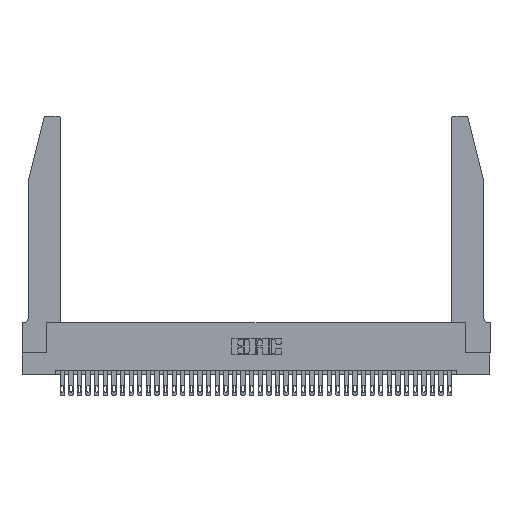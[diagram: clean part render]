
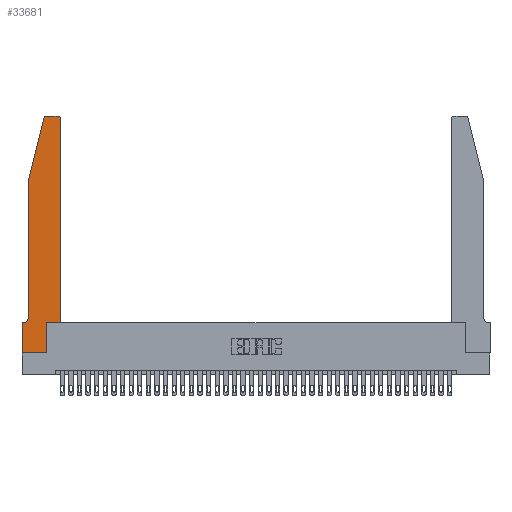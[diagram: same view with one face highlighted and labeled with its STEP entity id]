
A CAD part, top view. The second image highlights one B-rep face of the part: STEP entity #33681.
In plain terms, the highlighted planar face has unit normal (0, 0, 1).
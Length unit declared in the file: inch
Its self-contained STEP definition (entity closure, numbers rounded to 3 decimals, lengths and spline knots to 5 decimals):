
#63 = LINE ( 'NONE', #13842, #23939 ) ;
#73 = EDGE_CURVE ( 'NONE', #11095, #33877, #21612, .T. ) ;
#265 = CARTESIAN_POINT ( 'NONE',  ( 0.4505, 2.72, 0.37 ) ) ;
#416 = EDGE_CURVE ( 'NONE', #8961, #23256, #36718, .T. ) ;
#490 = VERTEX_POINT ( 'NONE', #5703 ) ;
#1253 = CARTESIAN_POINT ( 'NONE',  ( 0.0755, 0.42, 0.37 ) ) ;
#5703 = CARTESIAN_POINT ( 'NONE',  ( 0.4205, 2.75, 0.37 ) ) ;
#6117 = DIRECTION ( 'NONE',  ( 0., -1., 0. ) ) ;
#6192 = AXIS2_PLACEMENT_3D ( 'NONE', #17910, #31422, #35110 ) ;
#6345 = LINE ( 'NONE', #7668, #34552 ) ;
#7668 = CARTESIAN_POINT ( 'NONE',  ( 0.4505, 0.35, 0.37 ) ) ;
#7671 = CARTESIAN_POINT ( 'NONE',  ( 0.4205, 2.72, 0.37 ) ) ;
#7958 = CARTESIAN_POINT ( 'NONE',  ( 0., 0.35, 0.37 ) ) ;
#8218 = DIRECTION ( 'NONE',  ( 0., 0., 1. ) ) ;
#8357 = CARTESIAN_POINT ( 'NONE',  ( 0., 0., 0.37 ) ) ;
#8887 = CARTESIAN_POINT ( 'NONE',  ( 0.0755, 2., 0.37 ) ) ;
#8961 = VERTEX_POINT ( 'NONE', #23397 ) ;
#9012 = ORIENTED_EDGE ( 'NONE', *, *, #11675, .T. ) ;
#9973 = CARTESIAN_POINT ( 'NONE',  ( 0.0055, 0.35, 0.37 ) ) ;
#10136 = CARTESIAN_POINT ( 'NONE',  ( 0.4505, 0.35, 0.37 ) ) ;
#10383 = VERTEX_POINT ( 'NONE', #9973 ) ;
#10473 = ORIENTED_EDGE ( 'NONE', *, *, #33634, .T. ) ;
#10970 = DIRECTION ( 'NONE',  ( -0.239, -0.971, 0. ) ) ;
#11095 = VERTEX_POINT ( 'NONE', #32808 ) ;
#11608 = ORIENTED_EDGE ( 'NONE', *, *, #28059, .T. ) ;
#11675 = EDGE_CURVE ( 'NONE', #10383, #8961, #39729, .T. ) ;
#12038 = VERTEX_POINT ( 'NONE', #1253 ) ;
#12216 = EDGE_CURVE ( 'NONE', #490, #21823, #18283, .T. ) ;
#12367 = VECTOR ( 'NONE', #10970, 39.37008 ) ;
#12499 = ORIENTED_EDGE ( 'NONE', *, *, #33911, .T. ) ;
#12686 = LINE ( 'NONE', #8357, #39914 ) ;
#13035 = CIRCLE ( 'NONE', #6192, 0.07 ) ;
#13092 = DIRECTION ( 'NONE',  ( -1., 0., 0. ) ) ;
#13842 = CARTESIAN_POINT ( 'NONE',  ( 0.0755, 2., 0.37 ) ) ;
#14054 = CARTESIAN_POINT ( 'NONE',  ( 0., 0., 0.37 ) ) ;
#14530 = PLANE ( 'NONE',  #17660 ) ;
#14944 = VECTOR ( 'NONE', #13092, 39.37008 ) ;
#15720 = EDGE_LOOP ( 'NONE', ( #27569, #11608, #20144, #18434, #40113, #9012, #29407, #12499, #33056, #28661, #27659, #10473 ) ) ;
#16556 = CARTESIAN_POINT ( 'NONE',  ( 0.2865, 0.35, 0.37 ) ) ;
#16635 = LINE ( 'NONE', #16556, #20516 ) ;
#16700 = DIRECTION ( 'NONE',  ( 1., 0., 0. ) ) ;
#17660 = AXIS2_PLACEMENT_3D ( 'NONE', #7958, #8218, #20609 ) ;
#17910 = CARTESIAN_POINT ( 'NONE',  ( 0.0055, 0.42, 0.37 ) ) ;
#18283 = LINE ( 'NONE', #24377, #28432 ) ;
#18434 = ORIENTED_EDGE ( 'NONE', *, *, #18947, .T. ) ;
#18554 = CARTESIAN_POINT ( 'NONE',  ( 0.4505, 0.35, 0.37 ) ) ;
#18755 = DIRECTION ( 'NONE',  ( -1., 0., 0. ) ) ;
#18947 = EDGE_CURVE ( 'NONE', #33877, #12038, #63, .T. ) ;
#19023 = DIRECTION ( 'NONE',  ( 0., 0., 1. ) ) ;
#19150 = DIRECTION ( 'NONE',  ( 1., 0., 0. ) ) ;
#19734 = VERTEX_POINT ( 'NONE', #10136 ) ;
#20144 = ORIENTED_EDGE ( 'NONE', *, *, #73, .T. ) ;
#20476 = AXIS2_PLACEMENT_3D ( 'NONE', #7671, #38828, #29432 ) ;
#20516 = VECTOR ( 'NONE', #22787, 39.37008 ) ;
#20609 = DIRECTION ( 'NONE',  ( 1., 0., 0. ) ) ;
#21132 = AXIS2_PLACEMENT_3D ( 'NONE', #31755, #19023, #19150 ) ;
#21612 = LINE ( 'NONE', #36152, #12367 ) ;
#21823 = VERTEX_POINT ( 'NONE', #36470 ) ;
#22275 = CARTESIAN_POINT ( 'NONE',  ( 0.2865, 0.35, 0.37 ) ) ;
#22787 = DIRECTION ( 'NONE',  ( 0., 1., 0. ) ) ;
#22988 = CARTESIAN_POINT ( 'NONE',  ( 0.2865, 0., 0.37 ) ) ;
#23256 = VERTEX_POINT ( 'NONE', #33227 ) ;
#23397 = CARTESIAN_POINT ( 'NONE',  ( 0., 0.35, 0.37 ) ) ;
#23939 = VECTOR ( 'NONE', #6117, 39.37008 ) ;
#24105 = CIRCLE ( 'NONE', #21132, 0.03 ) ;
#24377 = CARTESIAN_POINT ( 'NONE',  ( 0.2605, 2.75, 0.37 ) ) ;
#24930 = VECTOR ( 'NONE', #28412, 39.37008 ) ;
#25309 = CIRCLE ( 'NONE', #20476, 0.03 ) ;
#25384 = VERTEX_POINT ( 'NONE', #22988 ) ;
#26394 = EDGE_CURVE ( 'NONE', #12038, #10383, #13035, .T. ) ;
#27569 = ORIENTED_EDGE ( 'NONE', *, *, #12216, .T. ) ;
#27659 = ORIENTED_EDGE ( 'NONE', *, *, #38008, .T. ) ;
#28059 = EDGE_CURVE ( 'NONE', #21823, #11095, #24105, .T. ) ;
#28412 = DIRECTION ( 'NONE',  ( 0., 1., 0. ) ) ;
#28432 = VECTOR ( 'NONE', #18755, 39.37008 ) ;
#28661 = ORIENTED_EDGE ( 'NONE', *, *, #30795, .T. ) ;
#29407 = ORIENTED_EDGE ( 'NONE', *, *, #416, .T. ) ;
#29432 = DIRECTION ( 'NONE',  ( 1., 0., 0. ) ) ;
#30786 = EDGE_CURVE ( 'NONE', #25384, #34609, #16635, .T. ) ;
#30795 = EDGE_CURVE ( 'NONE', #34609, #19734, #6345, .T. ) ;
#31422 = DIRECTION ( 'NONE',  ( 0., 0., -1. ) ) ;
#31534 = CARTESIAN_POINT ( 'NONE',  ( 0.0755, 0.35, 0.37 ) ) ;
#31755 = CARTESIAN_POINT ( 'NONE',  ( 0.284, 2.72, 0.37 ) ) ;
#32808 = CARTESIAN_POINT ( 'NONE',  ( 0.25487, 2.72718, 0.37 ) ) ;
#33056 = ORIENTED_EDGE ( 'NONE', *, *, #30786, .T. ) ;
#33227 = CARTESIAN_POINT ( 'NONE',  ( 0., 0., 0.37 ) ) ;
#33374 = DIRECTION ( 'NONE',  ( 1., 0., 0. ) ) ;
#33634 = EDGE_CURVE ( 'NONE', #33929, #490, #25309, .T. ) ;
#33681 = ADVANCED_FACE ( 'NONE', ( #35035 ), #14530, .T. ) ;
#33877 = VERTEX_POINT ( 'NONE', #8887 ) ;
#33911 = EDGE_CURVE ( 'NONE', #23256, #25384, #12686, .T. ) ;
#33929 = VERTEX_POINT ( 'NONE', #265 ) ;
#34552 = VECTOR ( 'NONE', #16700, 39.37008 ) ;
#34609 = VERTEX_POINT ( 'NONE', #22275 ) ;
#35035 = FACE_OUTER_BOUND ( 'NONE', #15720, .T. ) ;
#35110 = DIRECTION ( 'NONE',  ( -1., 0., 0. ) ) ;
#36152 = CARTESIAN_POINT ( 'NONE',  ( 0.0755, 2., 0.37 ) ) ;
#36470 = CARTESIAN_POINT ( 'NONE',  ( 0.284, 2.75, 0.37 ) ) ;
#36718 = LINE ( 'NONE', #14054, #40077 ) ;
#38008 = EDGE_CURVE ( 'NONE', #19734, #33929, #38557, .T. ) ;
#38471 = DIRECTION ( 'NONE',  ( 0., -1., 0. ) ) ;
#38557 = LINE ( 'NONE', #18554, #24930 ) ;
#38828 = DIRECTION ( 'NONE',  ( 0., 0., 1. ) ) ;
#39729 = LINE ( 'NONE', #31534, #14944 ) ;
#39914 = VECTOR ( 'NONE', #33374, 39.37008 ) ;
#40077 = VECTOR ( 'NONE', #38471, 39.37008 ) ;
#40113 = ORIENTED_EDGE ( 'NONE', *, *, #26394, .T. ) ;
